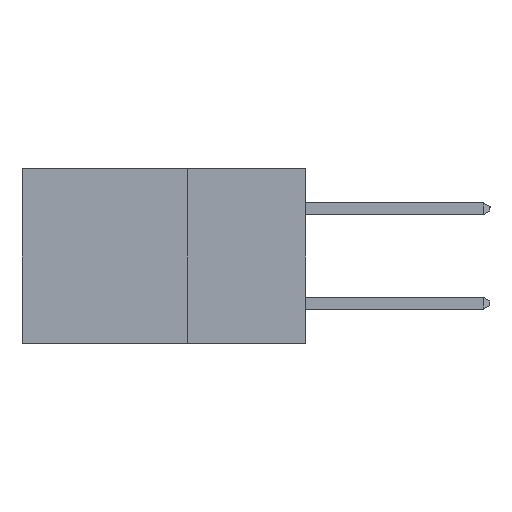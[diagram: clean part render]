
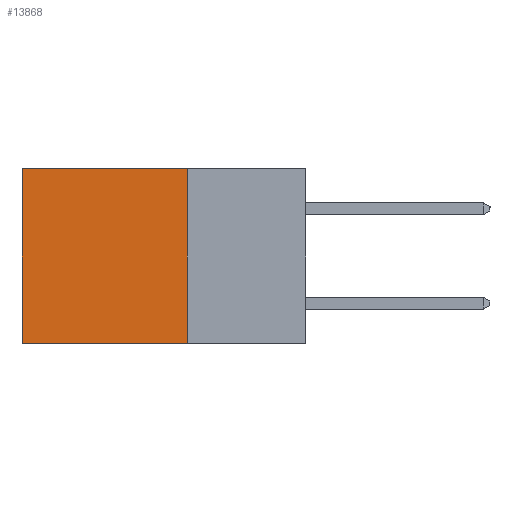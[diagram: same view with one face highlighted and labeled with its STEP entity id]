
A CAD part, left-side view. The second image highlights one B-rep face of the part: STEP entity #13868.
In plain terms, the highlighted planar face has unit normal (-1, 0, 0).
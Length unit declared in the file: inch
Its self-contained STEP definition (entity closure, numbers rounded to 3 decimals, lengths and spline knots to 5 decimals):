
#296 = DIRECTION ( 'NONE',  ( 0., 1., 0. ) ) ;
#311 = EDGE_CURVE ( 'NONE', #10553, #5953, #4323, .T. ) ;
#462 = DIRECTION ( 'NONE',  ( 0., 0., -1. ) ) ;
#789 = VECTOR ( 'NONE', #296, 39.37008 ) ;
#1195 = ORIENTED_EDGE ( 'NONE', *, *, #9266, .F. ) ;
#1433 = DIRECTION ( 'NONE',  ( 0., 0., -1. ) ) ;
#1454 = CARTESIAN_POINT ( 'NONE',  ( 0.2615, 0.25, 0. ) ) ;
#2596 = EDGE_CURVE ( 'NONE', #13080, #12077, #7924, .T. ) ;
#2632 = ORIENTED_EDGE ( 'NONE', *, *, #4287, .T. ) ;
#2817 = ORIENTED_EDGE ( 'NONE', *, *, #311, .T. ) ;
#3608 = CARTESIAN_POINT ( 'NONE',  ( 0.2615, 0.25, -0.37 ) ) ;
#3630 = CARTESIAN_POINT ( 'NONE',  ( 0.2615, 0.6, -0.37 ) ) ;
#4287 = EDGE_CURVE ( 'NONE', #5953, #12077, #16426, .T. ) ;
#4323 = LINE ( 'NONE', #14892, #789 ) ;
#4648 = CARTESIAN_POINT ( 'NONE',  ( 0.2615, 0.6, -0.37 ) ) ;
#5063 = DIRECTION ( 'NONE',  ( 0., 0., -1. ) ) ;
#5638 = CARTESIAN_POINT ( 'NONE',  ( 0.2615, 0.25, -0.37 ) ) ;
#5953 = VERTEX_POINT ( 'NONE', #14214 ) ;
#7053 = FACE_OUTER_BOUND ( 'NONE', #14145, .T. ) ;
#7219 = PLANE ( 'NONE',  #15195 ) ;
#7631 = ORIENTED_EDGE ( 'NONE', *, *, #2596, .F. ) ;
#7839 = VECTOR ( 'NONE', #462, 39.37008 ) ;
#7924 = LINE ( 'NONE', #14532, #13160 ) ;
#9266 = EDGE_CURVE ( 'NONE', #10553, #13080, #10891, .T. ) ;
#10553 = VERTEX_POINT ( 'NONE', #1454 ) ;
#10891 = LINE ( 'NONE', #5638, #12939 ) ;
#12077 = VERTEX_POINT ( 'NONE', #3630 ) ;
#12939 = VECTOR ( 'NONE', #1433, 39.37008 ) ;
#13080 = VERTEX_POINT ( 'NONE', #14893 ) ;
#13160 = VECTOR ( 'NONE', #15648, 39.37008 ) ;
#13868 = ADVANCED_FACE ( 'NONE', ( #7053 ), #7219, .F. ) ;
#14145 = EDGE_LOOP ( 'NONE', ( #2632, #7631, #1195, #2817 ) ) ;
#14214 = CARTESIAN_POINT ( 'NONE',  ( 0.2615, 0.6, 0. ) ) ;
#14532 = CARTESIAN_POINT ( 'NONE',  ( 0.2615, 0.25, -0.37 ) ) ;
#14892 = CARTESIAN_POINT ( 'NONE',  ( 0.2615, 0.25, 0. ) ) ;
#14893 = CARTESIAN_POINT ( 'NONE',  ( 0.2615, 0.25, -0.37 ) ) ;
#15195 = AXIS2_PLACEMENT_3D ( 'NONE', #3608, #16590, #5063 ) ;
#15648 = DIRECTION ( 'NONE',  ( 0., 1., 0. ) ) ;
#16426 = LINE ( 'NONE', #4648, #7839 ) ;
#16590 = DIRECTION ( 'NONE',  ( 1., 0., 0. ) ) ;
